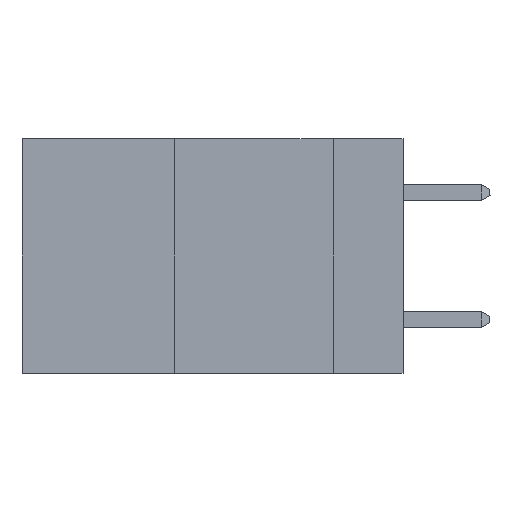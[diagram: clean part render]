
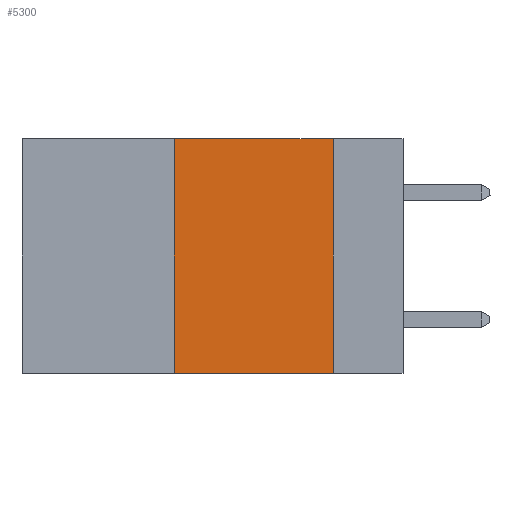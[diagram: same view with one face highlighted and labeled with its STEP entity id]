
A CAD part, left-side view. The second image highlights one B-rep face of the part: STEP entity #5300.
In plain terms, the highlighted planar face has unit normal (-1, 0, 0).
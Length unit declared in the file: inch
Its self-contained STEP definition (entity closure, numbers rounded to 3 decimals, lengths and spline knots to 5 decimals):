
#602 = VECTOR ( 'NONE', #32526, 39.37008 ) ;
#1686 = EDGE_CURVE ( 'NONE', #33572, #30147, #21514, .T. ) ;
#3902 = LINE ( 'NONE', #4103, #36384 ) ;
#4103 = CARTESIAN_POINT ( 'NONE',  ( 0., 0.6, 0. ) ) ;
#4915 = ORIENTED_EDGE ( 'NONE', *, *, #1686, .F. ) ;
#5017 = AXIS2_PLACEMENT_3D ( 'NONE', #6926, #29811, #36719 ) ;
#5129 = DIRECTION ( 'NONE',  ( 0., 0., -1. ) ) ;
#5300 = ADVANCED_FACE ( 'NONE', ( #7566 ), #26782, .F. ) ;
#5960 = ORIENTED_EDGE ( 'NONE', *, *, #8687, .T. ) ;
#6423 = CARTESIAN_POINT ( 'NONE',  ( 0., 0.6, -0.37 ) ) ;
#6926 = CARTESIAN_POINT ( 'NONE',  ( 0., 0.6, 0. ) ) ;
#7566 = FACE_OUTER_BOUND ( 'NONE', #41317, .T. ) ;
#8687 = EDGE_CURVE ( 'NONE', #9985, #30147, #25414, .T. ) ;
#9985 = VERTEX_POINT ( 'NONE', #20379 ) ;
#13491 = CARTESIAN_POINT ( 'NONE',  ( 0., 0.11, -0.37 ) ) ;
#16046 = ORIENTED_EDGE ( 'NONE', *, *, #31345, .F. ) ;
#17049 = DIRECTION ( 'NONE',  ( 0., -1., 0. ) ) ;
#19238 = CARTESIAN_POINT ( 'NONE',  ( 0., 0.36, 0. ) ) ;
#19351 = CARTESIAN_POINT ( 'NONE',  ( 0., 0.36, 0. ) ) ;
#20379 = CARTESIAN_POINT ( 'NONE',  ( 0., 0.36, -0.37 ) ) ;
#21514 = LINE ( 'NONE', #34689, #39476 ) ;
#24644 = VERTEX_POINT ( 'NONE', #19238 ) ;
#24905 = EDGE_CURVE ( 'NONE', #9985, #24644, #42274, .T. ) ;
#25414 = LINE ( 'NONE', #6423, #33831 ) ;
#26782 = PLANE ( 'NONE',  #5017 ) ;
#29811 = DIRECTION ( 'NONE',  ( 1., 0., 0. ) ) ;
#30147 = VERTEX_POINT ( 'NONE', #13491 ) ;
#31345 = EDGE_CURVE ( 'NONE', #24644, #33572, #3902, .T. ) ;
#32526 = DIRECTION ( 'NONE',  ( 0., 0., 1. ) ) ;
#33572 = VERTEX_POINT ( 'NONE', #39653 ) ;
#33831 = VECTOR ( 'NONE', #38582, 39.37008 ) ;
#34689 = CARTESIAN_POINT ( 'NONE',  ( 0., 0.11, 0. ) ) ;
#35067 = ORIENTED_EDGE ( 'NONE', *, *, #24905, .F. ) ;
#36384 = VECTOR ( 'NONE', #17049, 39.37008 ) ;
#36719 = DIRECTION ( 'NONE',  ( 0., 0., -1. ) ) ;
#38582 = DIRECTION ( 'NONE',  ( 0., -1., 0. ) ) ;
#39476 = VECTOR ( 'NONE', #5129, 39.37008 ) ;
#39653 = CARTESIAN_POINT ( 'NONE',  ( 0., 0.11, 0. ) ) ;
#41317 = EDGE_LOOP ( 'NONE', ( #4915, #16046, #35067, #5960 ) ) ;
#42274 = LINE ( 'NONE', #19351, #602 ) ;
